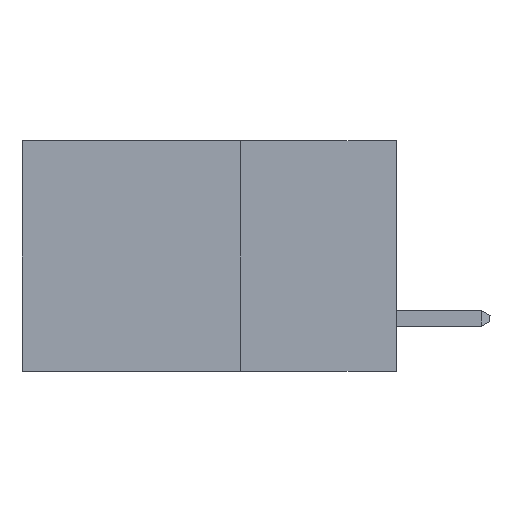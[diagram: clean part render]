
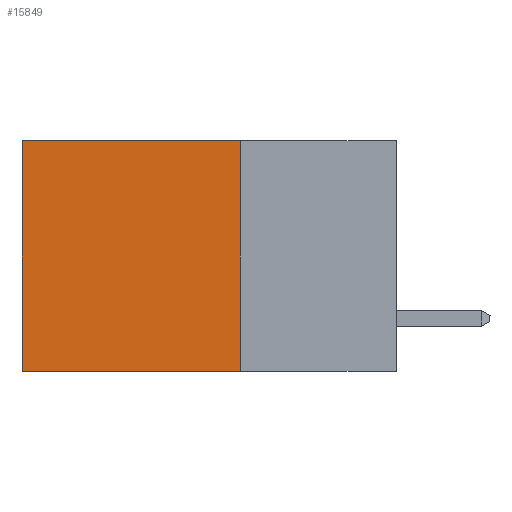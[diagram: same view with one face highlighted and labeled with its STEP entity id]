
A CAD part, left-side view. The second image highlights one B-rep face of the part: STEP entity #15849.
In plain terms, the highlighted planar face has unit normal (-1, 0, 0).
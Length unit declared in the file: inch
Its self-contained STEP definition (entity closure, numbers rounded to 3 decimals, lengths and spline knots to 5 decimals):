
#894 = DIRECTION ( 'NONE',  ( 0., 1., 0. ) ) ;
#2813 = CARTESIAN_POINT ( 'NONE',  ( 0.2615, 0.25, 0. ) ) ;
#4151 = VERTEX_POINT ( 'NONE', #22959 ) ;
#4412 = VERTEX_POINT ( 'NONE', #16656 ) ;
#4681 = EDGE_CURVE ( 'NONE', #4412, #16353, #6216, .T. ) ;
#6216 = LINE ( 'NONE', #10003, #15342 ) ;
#7131 = VECTOR ( 'NONE', #10332, 39.37008 ) ;
#7296 = CARTESIAN_POINT ( 'NONE',  ( 0.2615, 0.25, 0. ) ) ;
#7885 = CARTESIAN_POINT ( 'NONE',  ( 0.2615, 0.6, -0.37 ) ) ;
#8622 = DIRECTION ( 'NONE',  ( 0., 0., -1. ) ) ;
#8651 = CARTESIAN_POINT ( 'NONE',  ( 0.2615, 0.25, -0.37 ) ) ;
#9574 = EDGE_CURVE ( 'NONE', #4151, #16353, #15148, .T. ) ;
#9913 = EDGE_LOOP ( 'NONE', ( #11983, #17668, #19007, #21083 ) ) ;
#10003 = CARTESIAN_POINT ( 'NONE',  ( 0.2615, 0.25, -0.37 ) ) ;
#10332 = DIRECTION ( 'NONE',  ( 0., 0., -1. ) ) ;
#10463 = CARTESIAN_POINT ( 'NONE',  ( 0.2615, 0.6, -0.37 ) ) ;
#10932 = DIRECTION ( 'NONE',  ( 0., 1., 0. ) ) ;
#11983 = ORIENTED_EDGE ( 'NONE', *, *, #9574, .T. ) ;
#13216 = DIRECTION ( 'NONE',  ( 0., 0., -1. ) ) ;
#13256 = DIRECTION ( 'NONE',  ( 1., 0., 0. ) ) ;
#13314 = CARTESIAN_POINT ( 'NONE',  ( 0.2615, 0.25, -0.37 ) ) ;
#13330 = PLANE ( 'NONE',  #17959 ) ;
#13604 = FACE_OUTER_BOUND ( 'NONE', #9913, .T. ) ;
#15148 = LINE ( 'NONE', #10463, #7131 ) ;
#15342 = VECTOR ( 'NONE', #10932, 39.37008 ) ;
#15849 = ADVANCED_FACE ( 'NONE', ( #13604 ), #13330, .F. ) ;
#16273 = EDGE_CURVE ( 'NONE', #20544, #4412, #18756, .T. ) ;
#16281 = LINE ( 'NONE', #2813, #20308 ) ;
#16353 = VERTEX_POINT ( 'NONE', #7885 ) ;
#16656 = CARTESIAN_POINT ( 'NONE',  ( 0.2615, 0.25, -0.37 ) ) ;
#17128 = VECTOR ( 'NONE', #8622, 39.37008 ) ;
#17668 = ORIENTED_EDGE ( 'NONE', *, *, #4681, .F. ) ;
#17959 = AXIS2_PLACEMENT_3D ( 'NONE', #13314, #13256, #13216 ) ;
#18756 = LINE ( 'NONE', #8651, #17128 ) ;
#19007 = ORIENTED_EDGE ( 'NONE', *, *, #16273, .F. ) ;
#20308 = VECTOR ( 'NONE', #894, 39.37008 ) ;
#20544 = VERTEX_POINT ( 'NONE', #7296 ) ;
#21083 = ORIENTED_EDGE ( 'NONE', *, *, #21534, .T. ) ;
#21534 = EDGE_CURVE ( 'NONE', #20544, #4151, #16281, .T. ) ;
#22959 = CARTESIAN_POINT ( 'NONE',  ( 0.2615, 0.6, 0. ) ) ;
